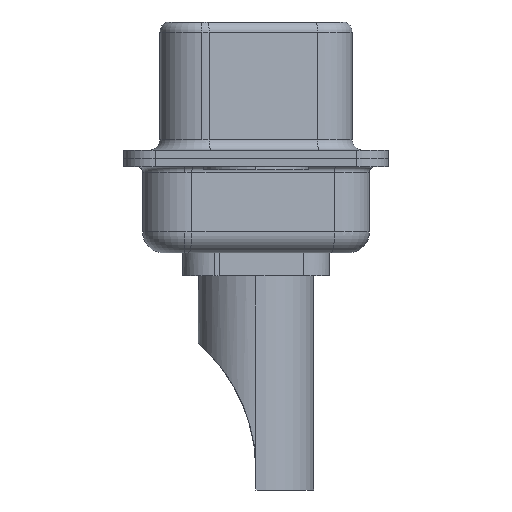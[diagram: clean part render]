
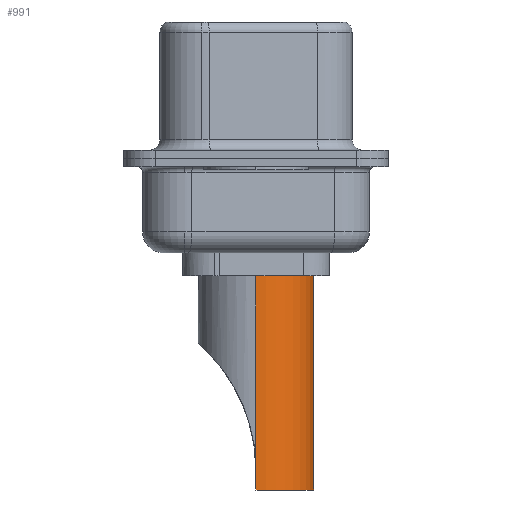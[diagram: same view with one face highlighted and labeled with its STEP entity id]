
A CAD part, left-side view. The second image highlights one B-rep face of the part: STEP entity #991.
In plain terms, the highlighted cylindrical face has radius 2.75 mm (diameter 5.5 mm), a partial arc.
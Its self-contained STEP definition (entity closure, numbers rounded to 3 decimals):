
#229 = EDGE_CURVE ( 'NONE', #11898, #1553, #9954, .T. ) ;
#287 = ORIENTED_EDGE ( 'NONE', *, *, #9760, .T. ) ;
#369 = CARTESIAN_POINT ( 'NONE',  ( -2.75, 0., 4.234 ) ) ;
#684 = ORIENTED_EDGE ( 'NONE', *, *, #4356, .F. ) ;
#991 = ADVANCED_FACE ( 'NONE', ( #1522 ), #9422, .T. ) ;
#1075 = CARTESIAN_POINT ( 'NONE',  ( -2.75, 0., -8.7 ) ) ;
#1371 = DIRECTION ( 'NONE',  ( 0., 0., -1. ) ) ;
#1522 = FACE_OUTER_BOUND ( 'NONE', #3404, .T. ) ;
#1526 = DIRECTION ( 'NONE',  ( 0., 0., 1. ) ) ;
#1553 = VERTEX_POINT ( 'NONE', #12308 ) ;
#1647 = EDGE_CURVE ( 'NONE', #9985, #9188, #5197, .T. ) ;
#2288 = DIRECTION ( 'NONE',  ( 1., 0., 0. ) ) ;
#2305 = DIRECTION ( 'NONE',  ( 0., 0., 1. ) ) ;
#2489 = VECTOR ( 'NONE', #6172, 1000. ) ;
#2679 = CARTESIAN_POINT ( 'NONE',  ( -2.75, 0., -8.7 ) ) ;
#2739 = VECTOR ( 'NONE', #1526, 1000. ) ;
#3404 = EDGE_LOOP ( 'NONE', ( #684, #9984, #8618, #8273, #287, #3835 ) ) ;
#3776 = CARTESIAN_POINT ( 'NONE',  ( 2.75, 0., -8.7 ) ) ;
#3835 = ORIENTED_EDGE ( 'NONE', *, *, #5956, .F. ) ;
#4237 = VECTOR ( 'NONE', #10582, 1000. ) ;
#4356 = EDGE_CURVE ( 'NONE', #9985, #9096, #11046, .T. ) ;
#4488 = CARTESIAN_POINT ( 'NONE',  ( 0., 0., 1.5 ) ) ;
#5197 = LINE ( 'NONE', #1075, #7711 ) ;
#5435 = AXIS2_PLACEMENT_3D ( 'NONE', #4488, #5653, #11651 ) ;
#5564 = LINE ( 'NONE', #9042, #2739 ) ;
#5653 = DIRECTION ( 'NONE',  ( 0., 0., 1. ) ) ;
#5956 = EDGE_CURVE ( 'NONE', #9096, #11995, #11903, .T. ) ;
#6172 = DIRECTION ( 'NONE',  ( 0., 0., 1. ) ) ;
#6309 = AXIS2_PLACEMENT_3D ( 'NONE', #7500, #2305, #2288 ) ;
#6490 = CARTESIAN_POINT ( 'NONE',  ( 2.75, 0., -7.764 ) ) ;
#6516 = EDGE_CURVE ( 'NONE', #9188, #1553, #13963, .T. ) ;
#6639 = DIRECTION ( 'NONE',  ( 0., 0., 1. ) ) ;
#6972 = DIRECTION ( 'NONE',  ( 1., 0., 0. ) ) ;
#7068 = CARTESIAN_POINT ( 'NONE',  ( 0., 0., 4.234 ) ) ;
#7170 = CARTESIAN_POINT ( 'NONE',  ( -2.75, 0., -7.764 ) ) ;
#7500 = CARTESIAN_POINT ( 'NONE',  ( 0., 0., -8.7 ) ) ;
#7711 = VECTOR ( 'NONE', #1371, 1000. ) ;
#8137 = AXIS2_PLACEMENT_3D ( 'NONE', #7068, #6639, #6972 ) ;
#8273 = ORIENTED_EDGE ( 'NONE', *, *, #229, .F. ) ;
#8618 = ORIENTED_EDGE ( 'NONE', *, *, #6516, .T. ) ;
#9042 = CARTESIAN_POINT ( 'NONE',  ( 2.75, 0., 4.234 ) ) ;
#9096 = VERTEX_POINT ( 'NONE', #10012 ) ;
#9188 = VERTEX_POINT ( 'NONE', #2679 ) ;
#9422 = CYLINDRICAL_SURFACE ( 'NONE', #8137, 2.75 ) ;
#9760 = EDGE_CURVE ( 'NONE', #11898, #11995, #5564, .T. ) ;
#9954 = LINE ( 'NONE', #3776, #4237 ) ;
#9984 = ORIENTED_EDGE ( 'NONE', *, *, #1647, .T. ) ;
#9985 = VERTEX_POINT ( 'NONE', #7170 ) ;
#10012 = CARTESIAN_POINT ( 'NONE',  ( -2.75, 0., 1.5 ) ) ;
#10582 = DIRECTION ( 'NONE',  ( 0., 0., -1. ) ) ;
#11046 = LINE ( 'NONE', #369, #2489 ) ;
#11651 = DIRECTION ( 'NONE',  ( 1., 0., 0. ) ) ;
#11898 = VERTEX_POINT ( 'NONE', #6490 ) ;
#11903 = CIRCLE ( 'NONE', #5435, 2.75 ) ;
#11995 = VERTEX_POINT ( 'NONE', #11999 ) ;
#11999 = CARTESIAN_POINT ( 'NONE',  ( 2.75, 0., 1.5 ) ) ;
#12308 = CARTESIAN_POINT ( 'NONE',  ( 2.75, 0., -8.7 ) ) ;
#13963 = CIRCLE ( 'NONE', #6309, 2.75 ) ;
